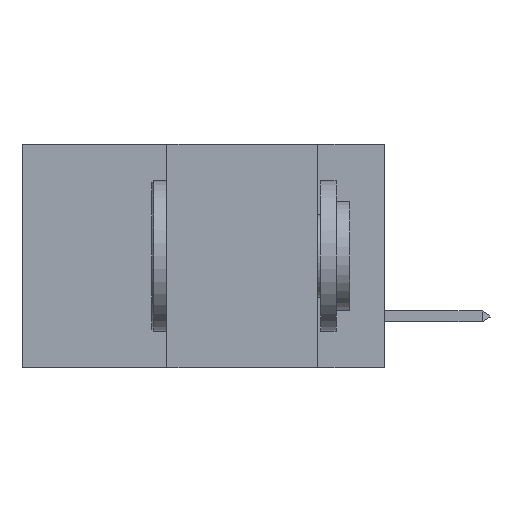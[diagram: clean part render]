
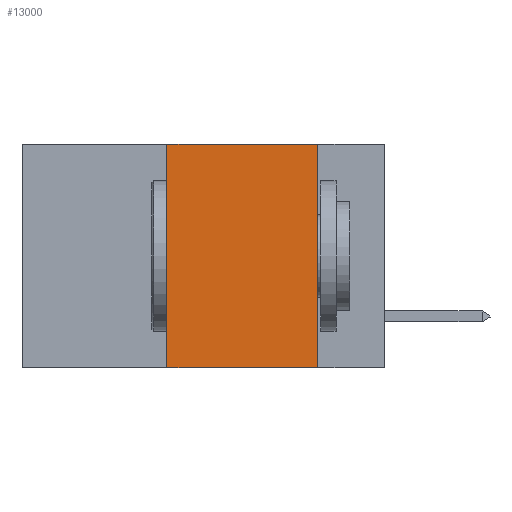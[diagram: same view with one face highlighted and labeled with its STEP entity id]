
A CAD part, left-side view. The second image highlights one B-rep face of the part: STEP entity #13000.
In plain terms, the highlighted planar face has unit normal (-1, 0, 0).
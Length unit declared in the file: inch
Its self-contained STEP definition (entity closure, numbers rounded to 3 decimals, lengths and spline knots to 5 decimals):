
#512 = LINE ( 'NONE', #17281, #15450 ) ;
#691 = ORIENTED_EDGE ( 'NONE', *, *, #4578, .F. ) ;
#1245 = PLANE ( 'NONE',  #5053 ) ;
#1646 = VERTEX_POINT ( 'NONE', #11788 ) ;
#1888 = DIRECTION ( 'NONE',  ( 1., 0., 0. ) ) ;
#3122 = LINE ( 'NONE', #7938, #18865 ) ;
#3449 = CARTESIAN_POINT ( 'NONE',  ( 0., 0.6, 0. ) ) ;
#4578 = EDGE_CURVE ( 'NONE', #1646, #14877, #13623, .T. ) ;
#5053 = AXIS2_PLACEMENT_3D ( 'NONE', #3449, #1888, #17127 ) ;
#6190 = CARTESIAN_POINT ( 'NONE',  ( 0., 0.11, 0. ) ) ;
#6404 = EDGE_LOOP ( 'NONE', ( #10584, #9395, #691, #14996 ) ) ;
#6568 = CARTESIAN_POINT ( 'NONE',  ( 0., 0.11, -0.37 ) ) ;
#7167 = VECTOR ( 'NONE', #22990, 39.37008 ) ;
#7938 = CARTESIAN_POINT ( 'NONE',  ( 0., 0.6, 0. ) ) ;
#9395 = ORIENTED_EDGE ( 'NONE', *, *, #20772, .F. ) ;
#10256 = EDGE_CURVE ( 'NONE', #1646, #17519, #512, .T. ) ;
#10584 = ORIENTED_EDGE ( 'NONE', *, *, #16925, .F. ) ;
#10950 = DIRECTION ( 'NONE',  ( 0., 0., -1. ) ) ;
#11645 = VECTOR ( 'NONE', #10950, 39.37008 ) ;
#11788 = CARTESIAN_POINT ( 'NONE',  ( 0., 0.36, -0.37 ) ) ;
#12617 = CARTESIAN_POINT ( 'NONE',  ( 0., 0.11, 0. ) ) ;
#13000 = ADVANCED_FACE ( 'NONE', ( #14140 ), #1245, .F. ) ;
#13623 = LINE ( 'NONE', #22830, #7167 ) ;
#14140 = FACE_OUTER_BOUND ( 'NONE', #6404, .T. ) ;
#14877 = VERTEX_POINT ( 'NONE', #20376 ) ;
#14996 = ORIENTED_EDGE ( 'NONE', *, *, #10256, .T. ) ;
#15450 = VECTOR ( 'NONE', #19044, 39.37008 ) ;
#16925 = EDGE_CURVE ( 'NONE', #17149, #17519, #18897, .T. ) ;
#17127 = DIRECTION ( 'NONE',  ( 0., 0., -1. ) ) ;
#17149 = VERTEX_POINT ( 'NONE', #6190 ) ;
#17281 = CARTESIAN_POINT ( 'NONE',  ( 0., 0.6, -0.37 ) ) ;
#17519 = VERTEX_POINT ( 'NONE', #6568 ) ;
#18865 = VECTOR ( 'NONE', #20316, 39.37008 ) ;
#18897 = LINE ( 'NONE', #12617, #11645 ) ;
#19044 = DIRECTION ( 'NONE',  ( 0., -1., 0. ) ) ;
#20316 = DIRECTION ( 'NONE',  ( 0., -1., 0. ) ) ;
#20376 = CARTESIAN_POINT ( 'NONE',  ( 0., 0.36, 0. ) ) ;
#20772 = EDGE_CURVE ( 'NONE', #14877, #17149, #3122, .T. ) ;
#22830 = CARTESIAN_POINT ( 'NONE',  ( 0., 0.36, 0. ) ) ;
#22990 = DIRECTION ( 'NONE',  ( 0., 0., 1. ) ) ;
